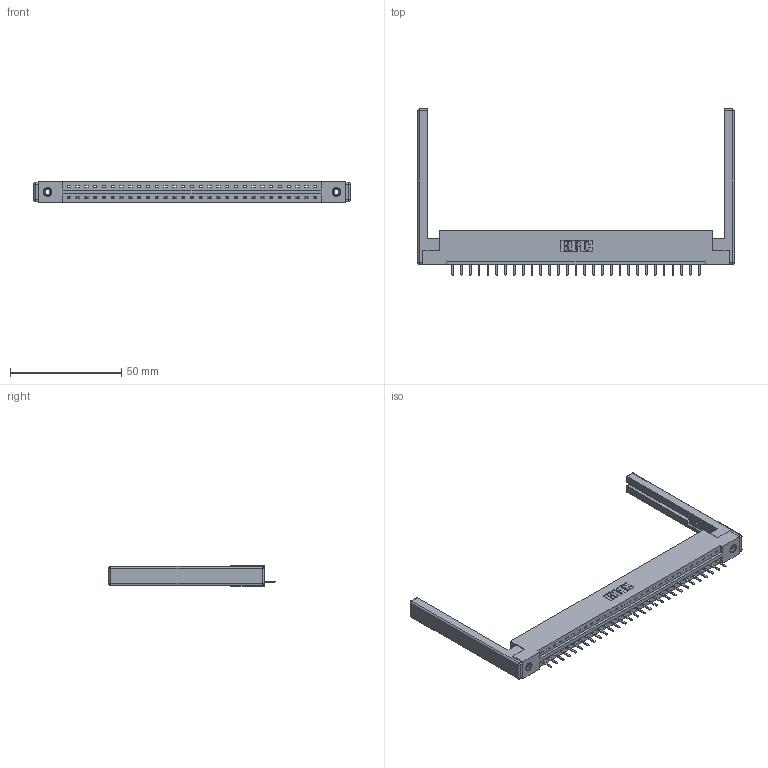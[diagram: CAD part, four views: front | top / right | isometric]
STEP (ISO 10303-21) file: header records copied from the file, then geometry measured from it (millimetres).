
FILE_DESCRIPTION (( 'STEP AP203' ), '1' );
FILE_NAME ('387-029-520-168.STEP', '2019-10-03T16:44:18', ( '' ), ( '' ), 'SwSTEP 2.0', 'SolidWorks 2016', '' );
FILE_SCHEMA (( 'CONFIG_CONTROL_DESIGN' ));
Length unit declared in the file: inch
Products named in the file (5): 345-292-001_345-293-120; 337 Part_Flush Mounting Lugs - 0.156 Dia-TI; 387-029-520-168; 307-220-068; 345-250-001_345-250-001-102
Assembly tree (34 placements, depth 2):
  387-029-520-168
    337 Part_Flush Mounting Lugs - 0.156 Dia-TI
    345-292-001_345-293-120  x29
    345-250-001_345-250-001-102  x2
    307-220-068  x2
Bounding box: 142.34 x 74.76 x 9.4 mm (x, y, z)
Volume: 18939.1 mm3; surface area: 18753.4 mm2
Topology: 34 solids, 34 shells, 2182 faces, 6385 edges, 4158 vertices
Faces by surface type: plane 1550, cylinder 608, cone 12, sphere 8, torus 4
Entity records: 26112 total; most frequent: CARTESIAN_POINT 4514, ORIENTED_EDGE 4456, DIRECTION 3888, EDGE_CURVE 2228, VECTOR 2046, LINE 2046, VERTEX_POINT 1474, AXIS2_PLACEMENT_3D 921
